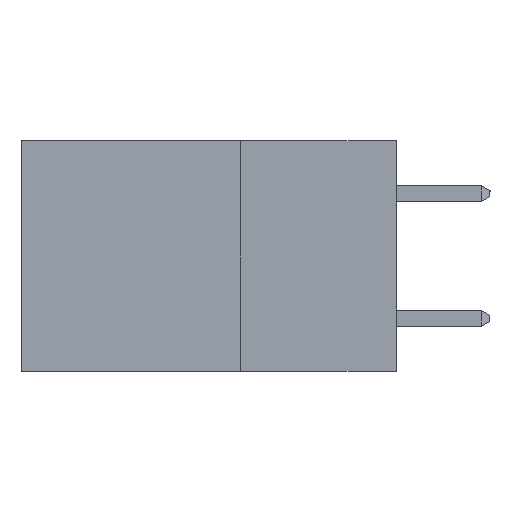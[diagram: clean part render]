
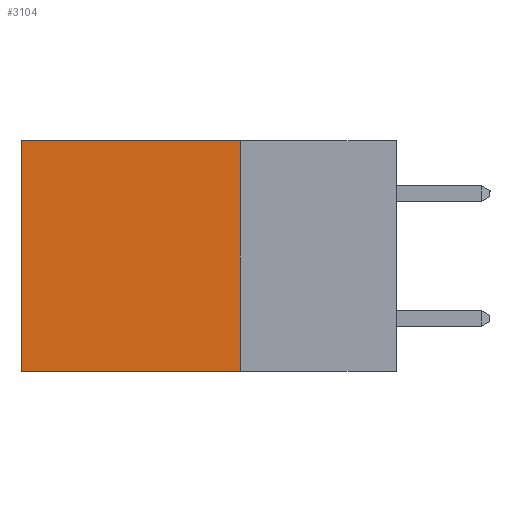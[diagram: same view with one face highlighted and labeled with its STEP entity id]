
A CAD part, left-side view. The second image highlights one B-rep face of the part: STEP entity #3104.
In plain terms, the highlighted planar face has unit normal (-1, 0, 0).
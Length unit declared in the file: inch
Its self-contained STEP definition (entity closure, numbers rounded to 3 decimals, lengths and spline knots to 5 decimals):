
#105 = DIRECTION ( 'NONE',  ( 0., 1., 0. ) ) ;
#453 = VECTOR ( 'NONE', #11024, 39.37008 ) ;
#581 = VERTEX_POINT ( 'NONE', #9488 ) ;
#1028 = VERTEX_POINT ( 'NONE', #7156 ) ;
#1131 = EDGE_LOOP ( 'NONE', ( #3761, #13526, #6232, #2949 ) ) ;
#1191 = DIRECTION ( 'NONE',  ( 1., 0., 0. ) ) ;
#1262 = CARTESIAN_POINT ( 'NONE',  ( 0.2615, 0.25, 0. ) ) ;
#1348 = CARTESIAN_POINT ( 'NONE',  ( 0.2615, 0.6, -0.37 ) ) ;
#2761 = AXIS2_PLACEMENT_3D ( 'NONE', #6895, #1191, #6821 ) ;
#2949 = ORIENTED_EDGE ( 'NONE', *, *, #8265, .T. ) ;
#3104 = ADVANCED_FACE ( 'NONE', ( #11552 ), #5945, .F. ) ;
#3761 = ORIENTED_EDGE ( 'NONE', *, *, #8710, .T. ) ;
#5044 = VERTEX_POINT ( 'NONE', #8490 ) ;
#5277 = LINE ( 'NONE', #14778, #453 ) ;
#5611 = VECTOR ( 'NONE', #6939, 39.37008 ) ;
#5945 = PLANE ( 'NONE',  #2761 ) ;
#6028 = VERTEX_POINT ( 'NONE', #1348 ) ;
#6054 = VECTOR ( 'NONE', #10294, 39.37008 ) ;
#6232 = ORIENTED_EDGE ( 'NONE', *, *, #12538, .F. ) ;
#6732 = LINE ( 'NONE', #10368, #6054 ) ;
#6821 = DIRECTION ( 'NONE',  ( 0., 0., -1. ) ) ;
#6895 = CARTESIAN_POINT ( 'NONE',  ( 0.2615, 0.25, -0.37 ) ) ;
#6917 = EDGE_CURVE ( 'NONE', #581, #6028, #5277, .T. ) ;
#6939 = DIRECTION ( 'NONE',  ( 0., 0., -1. ) ) ;
#7156 = CARTESIAN_POINT ( 'NONE',  ( 0.2615, 0.25, 0. ) ) ;
#8265 = EDGE_CURVE ( 'NONE', #1028, #5044, #8451, .T. ) ;
#8451 = LINE ( 'NONE', #1262, #10742 ) ;
#8490 = CARTESIAN_POINT ( 'NONE',  ( 0.2615, 0.6, 0. ) ) ;
#8710 = EDGE_CURVE ( 'NONE', #5044, #6028, #6732, .T. ) ;
#9488 = CARTESIAN_POINT ( 'NONE',  ( 0.2615, 0.25, -0.37 ) ) ;
#10294 = DIRECTION ( 'NONE',  ( 0., 0., -1. ) ) ;
#10368 = CARTESIAN_POINT ( 'NONE',  ( 0.2615, 0.6, -0.37 ) ) ;
#10742 = VECTOR ( 'NONE', #105, 39.37008 ) ;
#11024 = DIRECTION ( 'NONE',  ( 0., 1., 0. ) ) ;
#11552 = FACE_OUTER_BOUND ( 'NONE', #1131, .T. ) ;
#11597 = CARTESIAN_POINT ( 'NONE',  ( 0.2615, 0.25, -0.37 ) ) ;
#12538 = EDGE_CURVE ( 'NONE', #1028, #581, #12840, .T. ) ;
#12840 = LINE ( 'NONE', #11597, #5611 ) ;
#13526 = ORIENTED_EDGE ( 'NONE', *, *, #6917, .F. ) ;
#14778 = CARTESIAN_POINT ( 'NONE',  ( 0.2615, 0.25, -0.37 ) ) ;
